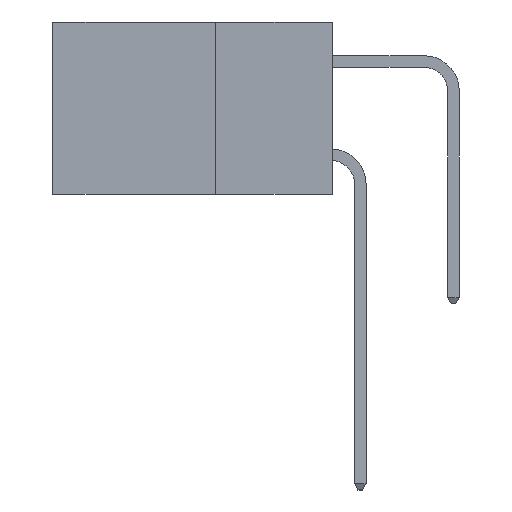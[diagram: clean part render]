
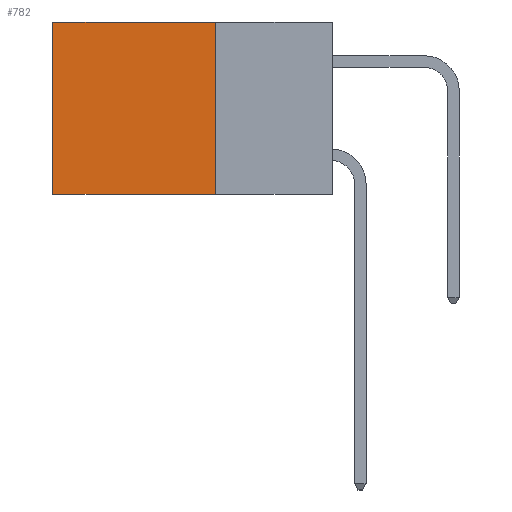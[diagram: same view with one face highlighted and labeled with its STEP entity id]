
A CAD part, left-side view. The second image highlights one B-rep face of the part: STEP entity #782.
In plain terms, the highlighted planar face has unit normal (-1, 0, 0).
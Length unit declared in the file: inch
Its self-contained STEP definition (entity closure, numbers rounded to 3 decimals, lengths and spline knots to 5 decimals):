
#601 = VECTOR ( 'NONE', #11901, 39.37008 ) ;
#782 = ADVANCED_FACE ( 'NONE', ( #5031 ), #14954, .F. ) ;
#1900 = VERTEX_POINT ( 'NONE', #11031 ) ;
#2402 = CARTESIAN_POINT ( 'NONE',  ( 0.2615, 0.25, -0.37 ) ) ;
#2526 = DIRECTION ( 'NONE',  ( 0., 1., 0. ) ) ;
#2598 = VERTEX_POINT ( 'NONE', #2725 ) ;
#2725 = CARTESIAN_POINT ( 'NONE',  ( 0.2615, 0.6, 0. ) ) ;
#2906 = ORIENTED_EDGE ( 'NONE', *, *, #12507, .F. ) ;
#3337 = CARTESIAN_POINT ( 'NONE',  ( 0.2615, 0.25, -0.37 ) ) ;
#3419 = DIRECTION ( 'NONE',  ( 1., 0., 0. ) ) ;
#4781 = DIRECTION ( 'NONE',  ( 0., 0., -1. ) ) ;
#5031 = FACE_OUTER_BOUND ( 'NONE', #8695, .T. ) ;
#5735 = CARTESIAN_POINT ( 'NONE',  ( 0.2615, 0.25, 0. ) ) ;
#5791 = CARTESIAN_POINT ( 'NONE',  ( 0.2615, 0.6, -0.37 ) ) ;
#5855 = DIRECTION ( 'NONE',  ( 0., 1., 0. ) ) ;
#6218 = ORIENTED_EDGE ( 'NONE', *, *, #14551, .F. ) ;
#8137 = CARTESIAN_POINT ( 'NONE',  ( 0.2615, 0.25, -0.37 ) ) ;
#8312 = VECTOR ( 'NONE', #5855, 39.37008 ) ;
#8695 = EDGE_LOOP ( 'NONE', ( #15092, #2906, #6218, #12680 ) ) ;
#8702 = VERTEX_POINT ( 'NONE', #14720 ) ;
#9010 = VECTOR ( 'NONE', #11748, 39.37008 ) ;
#9442 = VECTOR ( 'NONE', #2526, 39.37008 ) ;
#9444 = LINE ( 'NONE', #5735, #8312 ) ;
#10163 = CARTESIAN_POINT ( 'NONE',  ( 0.2615, 0.25, -0.37 ) ) ;
#10700 = LINE ( 'NONE', #5791, #601 ) ;
#11031 = CARTESIAN_POINT ( 'NONE',  ( 0.2615, 0.25, 0. ) ) ;
#11748 = DIRECTION ( 'NONE',  ( 0., 0., -1. ) ) ;
#11901 = DIRECTION ( 'NONE',  ( 0., 0., -1. ) ) ;
#12009 = EDGE_CURVE ( 'NONE', #1900, #2598, #9444, .T. ) ;
#12371 = VERTEX_POINT ( 'NONE', #3337 ) ;
#12507 = EDGE_CURVE ( 'NONE', #12371, #8702, #12560, .T. ) ;
#12515 = LINE ( 'NONE', #8137, #9010 ) ;
#12560 = LINE ( 'NONE', #2402, #9442 ) ;
#12680 = ORIENTED_EDGE ( 'NONE', *, *, #12009, .T. ) ;
#14551 = EDGE_CURVE ( 'NONE', #1900, #12371, #12515, .T. ) ;
#14656 = EDGE_CURVE ( 'NONE', #2598, #8702, #10700, .T. ) ;
#14720 = CARTESIAN_POINT ( 'NONE',  ( 0.2615, 0.6, -0.37 ) ) ;
#14954 = PLANE ( 'NONE',  #15476 ) ;
#15092 = ORIENTED_EDGE ( 'NONE', *, *, #14656, .T. ) ;
#15476 = AXIS2_PLACEMENT_3D ( 'NONE', #10163, #3419, #4781 ) ;
